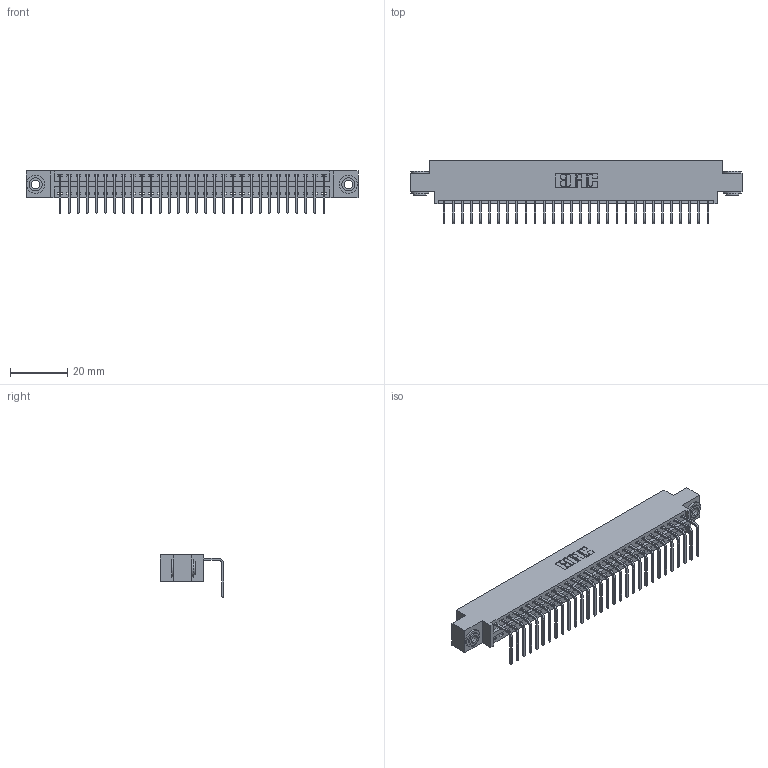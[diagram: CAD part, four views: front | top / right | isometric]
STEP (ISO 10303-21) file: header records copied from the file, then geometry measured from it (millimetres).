
FILE_DESCRIPTION (( 'STEP AP203' ), '1' );
FILE_NAME ('396-030-558-603.STEP', '2019-11-01T06:56:05', ( '' ), ( '' ), 'SwSTEP 2.0', 'SolidWorks 2016', '' );
FILE_SCHEMA (( 'CONFIG_CONTROL_DESIGN' ));
Length unit declared in the file: inch
Products named in the file (4): 345-250-002_345-250-002-102; 396-030-558-603; 346 Part_0.170 Offset - 0.156 Dia-TH; 345-292-001_558 Tail - 2
Assembly tree (33 placements, depth 2):
  396-030-558-603
    346 Part_0.170 Offset - 0.156 Dia-TH
    345-292-001_558 Tail - 2  x30
    345-250-002_345-250-002-102  x2
Bounding box: 115.82 x 22.16 x 14.73 mm (x, y, z)
Volume: 10969 mm3; surface area: 14556.1 mm2
Topology: 33 solids, 33 shells, 1964 faces, 5877 edges, 3874 vertices
Faces by surface type: plane 1350, cylinder 606, cone 8
Entity records: 21100 total; most frequent: CARTESIAN_POINT 3601, ORIENTED_EDGE 3558, DIRECTION 3221, EDGE_CURVE 1779, LINE 1503, VECTOR 1503, VERTEX_POINT 1182, AXIS2_PLACEMENT_3D 859
